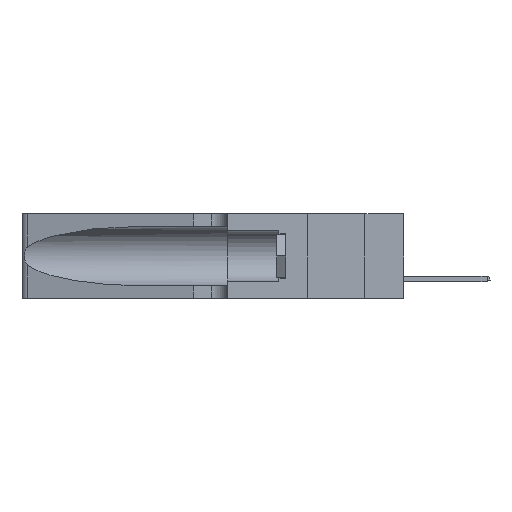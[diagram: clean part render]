
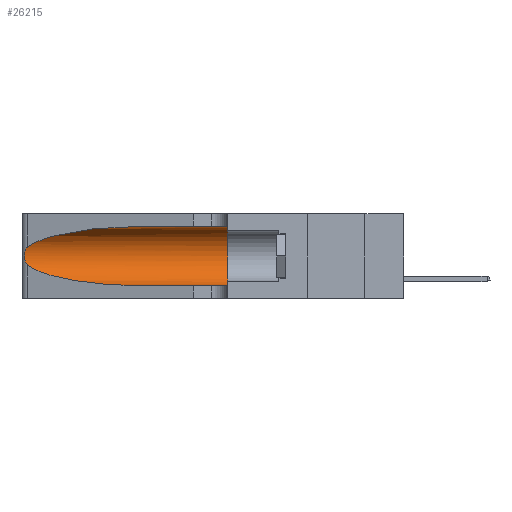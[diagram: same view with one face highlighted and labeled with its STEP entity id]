
A CAD part, left-side view. The second image highlights one B-rep face of the part: STEP entity #26215.
In plain terms, the highlighted cylindrical face has radius 3.308 mm (diameter 6.617 mm), a partial arc.
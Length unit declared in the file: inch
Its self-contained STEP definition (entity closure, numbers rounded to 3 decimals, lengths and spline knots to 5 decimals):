
#650 = EDGE_CURVE ( 'NONE', #44700, #46243, #19876, .T. ) ;
#724 = DIRECTION ( 'NONE',  ( 0., -1., 0. ) ) ;
#1289 = CYLINDRICAL_SURFACE ( 'NONE', #1674, 0.13025 ) ;
#1463 = CARTESIAN_POINT ( 'NONE',  ( 0.25639, 1.23184, 0.21858 ) ) ;
#1523 = LINE ( 'NONE', #49946, #23059 ) ;
#1667 = CARTESIAN_POINT ( 'NONE',  ( 0.25787, 1.23484, 0.2124 ) ) ;
#1674 = AXIS2_PLACEMENT_3D ( 'NONE', #17739, #25681, #33185 ) ;
#1960 = VERTEX_POINT ( 'NONE', #37145 ) ;
#2071 = CARTESIAN_POINT ( 'NONE',  ( 0.26018, 1.23835, 0.19895 ) ) ;
#3189 = ORIENTED_EDGE ( 'NONE', *, *, #25084, .T. ) ;
#3724 = VERTEX_POINT ( 'NONE', #7204 ) ;
#4277 = CARTESIAN_POINT ( 'NONE',  ( 0.18966, 0.96281, 0.05475 ) ) ;
#4533 = B_SPLINE_CURVE_WITH_KNOTS ( 'NONE', 3,
 ( #16334, #28472, #1463, #1667, #36916, #2071, #38531, #48287, #11767, #32600, #32514, #15521, #19905, #31854 ),
 .UNSPECIFIED., .F., .F.,
 ( 4, 2, 2, 2, 2, 2, 4 ),
 ( 0., 0.00027, 0.00053, 0.00107, 0.0016, 0.00187, 0.00214 ),
 .UNSPECIFIED. ) ;
#5286 = CARTESIAN_POINT ( 'NONE',  ( 0.1305, 0.72297, 0.31525 ) ) ;
#5866 = CARTESIAN_POINT ( 'NONE',  ( 0.25487, 1.22718, 0.22369 ) ) ;
#7204 = CARTESIAN_POINT ( 'NONE',  ( 0.1305, 0.35, 0.05475 ) ) ;
#8117 = CARTESIAN_POINT ( 'NONE',  ( 0.2373, 1.15595, 0.08982 ) ) ;
#8202 = CIRCLE ( 'NONE', #32534, 0.13025 ) ;
#8680 = ORIENTED_EDGE ( 'NONE', *, *, #15362, .T. ) ;
#8826 = DIRECTION ( 'NONE',  ( 0., 0., 1. ) ) ;
#11767 = CARTESIAN_POINT ( 'NONE',  ( 0.26017, 1.23833, 0.17102 ) ) ;
#11952 = ORIENTED_EDGE ( 'NONE', *, *, #38942, .T. ) ;
#15084 = VERTEX_POINT ( 'NONE', #39618 ) ;
#15362 = EDGE_CURVE ( 'NONE', #44700, #39231, #49382, .T. ) ;
#15521 = CARTESIAN_POINT ( 'NONE',  ( 0.25639, 1.23186, 0.15144 ) ) ;
#16165 = CARTESIAN_POINT ( 'NONE',  ( 0.1305, 0.72297, 0.05475 ) ) ;
#16334 = CARTESIAN_POINT ( 'NONE',  ( 0.25487, 1.22718, 0.22369 ) ) ;
#17739 = CARTESIAN_POINT ( 'NONE',  ( 0.1305, 1.61858, 0.185 ) ) ;
#18337 = CARTESIAN_POINT ( 'NONE',  ( 0.18966, 0.96281, 0.31525 ) ) ;
#19103 = EDGE_LOOP ( 'NONE', ( #8680, #3189, #19801, #11952, #32624, #50014 ) ) ;
#19801 = ORIENTED_EDGE ( 'NONE', *, *, #49334, .T. ) ;
#19876 = LINE ( 'NONE', #20796, #26127 ) ;
#19905 = CARTESIAN_POINT ( 'NONE',  ( 0.25555, 1.22993, 0.14849 ) ) ;
#20796 = CARTESIAN_POINT ( 'NONE',  ( 0.1305, 1.61858, 0.31525 ) ) ;
#23059 = VECTOR ( 'NONE', #49211, 39.37008 ) ;
#24623 = CARTESIAN_POINT ( 'NONE',  ( 0.25487, 1.22718, 0.14631 ) ) ;
#25084 = EDGE_CURVE ( 'NONE', #39231, #1960, #4533, .T. ) ;
#25681 = DIRECTION ( 'NONE',  ( 0., -1., 0. ) ) ;
#25890 = CARTESIAN_POINT ( 'NONE',  ( 0.1305, 0.72297, 0.31525 ) ) ;
#26127 = VECTOR ( 'NONE', #724, 39.37008 ) ;
#26215 = ADVANCED_FACE ( 'NONE', ( #31606 ), #1289, .F. ) ;
#26459 = CARTESIAN_POINT ( 'NONE',  ( 0.2373, 1.15595, 0.28018 ) ) ;
#28472 = CARTESIAN_POINT ( 'NONE',  ( 0.25555, 1.22994, 0.2215 ) ) ;
#28673 =( BOUNDED_CURVE ( )  B_SPLINE_CURVE ( 3, ( #24623, #8117, #4277, #16165 ),
 .UNSPECIFIED., .F., .F. ) 
 B_SPLINE_CURVE_WITH_KNOTS ( ( 4, 4 ),
 ( 3.44316, 4.71239 ),
 .UNSPECIFIED. ) 
 CURVE ( )  GEOMETRIC_REPRESENTATION_ITEM ( )  RATIONAL_B_SPLINE_CURVE ( ( 1., 0.87, 0.87, 1. ) ) 
 REPRESENTATION_ITEM ( '' )  );
#31200 = CARTESIAN_POINT ( 'NONE',  ( 0.1305, 0.35, 0.31525 ) ) ;
#31606 = FACE_OUTER_BOUND ( 'NONE', #19103, .T. ) ;
#31854 = CARTESIAN_POINT ( 'NONE',  ( 0.25487, 1.22718, 0.14631 ) ) ;
#32514 = CARTESIAN_POINT ( 'NONE',  ( 0.25789, 1.23486, 0.15765 ) ) ;
#32534 = AXIS2_PLACEMENT_3D ( 'NONE', #36687, #41171, #8826 ) ;
#32600 = CARTESIAN_POINT ( 'NONE',  ( 0.25856, 1.23593, 0.16098 ) ) ;
#32624 = ORIENTED_EDGE ( 'NONE', *, *, #42018, .F. ) ;
#33185 = DIRECTION ( 'NONE',  ( 0., 0., -1. ) ) ;
#36687 = CARTESIAN_POINT ( 'NONE',  ( 0.1305, 0.35, 0.185 ) ) ;
#36916 = CARTESIAN_POINT ( 'NONE',  ( 0.25854, 1.2359, 0.20912 ) ) ;
#37145 = CARTESIAN_POINT ( 'NONE',  ( 0.25487, 1.22718, 0.14631 ) ) ;
#38531 = CARTESIAN_POINT ( 'NONE',  ( 0.26075, 1.23896, 0.19203 ) ) ;
#38942 = EDGE_CURVE ( 'NONE', #15084, #3724, #1523, .T. ) ;
#39231 = VERTEX_POINT ( 'NONE', #43687 ) ;
#39618 = CARTESIAN_POINT ( 'NONE',  ( 0.1305, 0.72297, 0.05475 ) ) ;
#41171 = DIRECTION ( 'NONE',  ( 0., 1., 0. ) ) ;
#42018 = EDGE_CURVE ( 'NONE', #46243, #3724, #8202, .T. ) ;
#43687 = CARTESIAN_POINT ( 'NONE',  ( 0.25487, 1.22718, 0.22369 ) ) ;
#44700 = VERTEX_POINT ( 'NONE', #5286 ) ;
#46243 = VERTEX_POINT ( 'NONE', #31200 ) ;
#48287 = CARTESIAN_POINT ( 'NONE',  ( 0.26075, 1.23896, 0.178 ) ) ;
#49211 = DIRECTION ( 'NONE',  ( 0., -1., 0. ) ) ;
#49334 = EDGE_CURVE ( 'NONE', #1960, #15084, #28673, .T. ) ;
#49382 =( BOUNDED_CURVE ( )  B_SPLINE_CURVE ( 3, ( #25890, #18337, #26459, #5866 ),
 .UNSPECIFIED., .F., .T. ) 
 B_SPLINE_CURVE_WITH_KNOTS ( ( 4, 4 ),
 ( 1.5708, 2.84003 ),
 .UNSPECIFIED. ) 
 CURVE ( )  GEOMETRIC_REPRESENTATION_ITEM ( )  RATIONAL_B_SPLINE_CURVE ( ( 1., 0.87, 0.87, 1. ) ) 
 REPRESENTATION_ITEM ( '' )  );
#49946 = CARTESIAN_POINT ( 'NONE',  ( 0.1305, 1.61858, 0.05475 ) ) ;
#50014 = ORIENTED_EDGE ( 'NONE', *, *, #650, .F. ) ;
